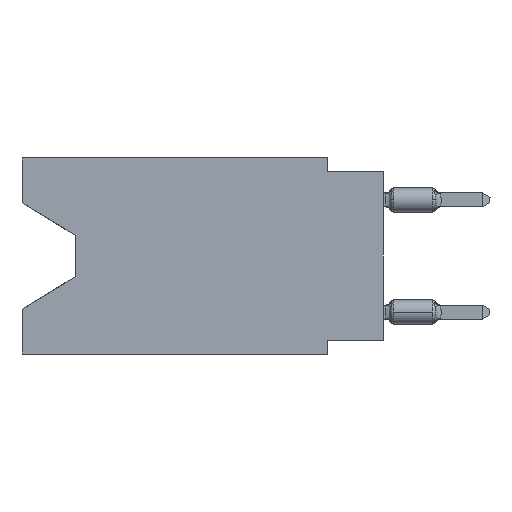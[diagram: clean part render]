
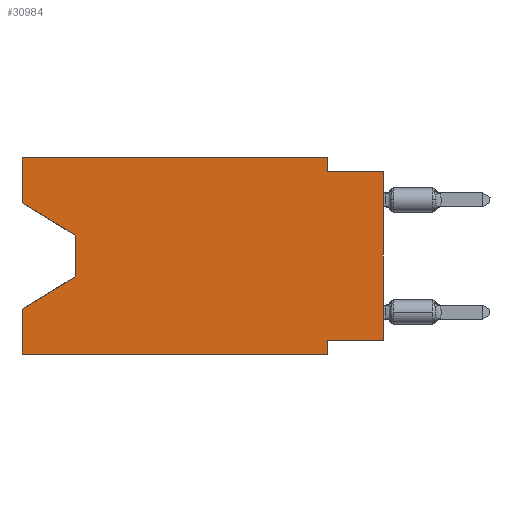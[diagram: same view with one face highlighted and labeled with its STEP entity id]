
A CAD part, left-side view. The second image highlights one B-rep face of the part: STEP entity #30984.
In plain terms, the highlighted planar face has unit normal (-1, 0, 0).
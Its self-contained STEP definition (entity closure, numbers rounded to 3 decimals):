
#1285 = VERTEX_POINT ( 'NONE', #12462 ) ;
#3430 = CARTESIAN_POINT ( 'NONE',  ( 0., 16.383, 0. ) ) ;
#3549 = VERTEX_POINT ( 'NONE', #6549 ) ;
#4236 = VERTEX_POINT ( 'NONE', #45789 ) ;
#4736 = DIRECTION ( 'NONE',  ( 0., -1., 0. ) ) ;
#6002 = CARTESIAN_POINT ( 'NONE',  ( 0., 16.383, 0. ) ) ;
#6549 = CARTESIAN_POINT ( 'NONE',  ( 0., 2.54, -8.89 ) ) ;
#6741 = ORIENTED_EDGE ( 'NONE', *, *, #22903, .F. ) ;
#6916 = LINE ( 'NONE', #33913, #56419 ) ;
#7163 = ORIENTED_EDGE ( 'NONE', *, *, #11240, .T. ) ;
#7805 = EDGE_CURVE ( 'NONE', #14312, #40535, #52317, .T. ) ;
#7838 = DIRECTION ( 'NONE',  ( 0., -1., 0. ) ) ;
#7940 = VECTOR ( 'NONE', #47661, 1000. ) ;
#7966 = ORIENTED_EDGE ( 'NONE', *, *, #21725, .T. ) ;
#8122 = CARTESIAN_POINT ( 'NONE',  ( 0., 16.383, -8.89 ) ) ;
#8151 = VECTOR ( 'NONE', #15307, 1000. ) ;
#8404 = ORIENTED_EDGE ( 'NONE', *, *, #32919, .F. ) ;
#9423 = DIRECTION ( 'NONE',  ( 0., 0., -1. ) ) ;
#9723 = LINE ( 'NONE', #51548, #49318 ) ;
#10751 = DIRECTION ( 'NONE',  ( 1., 0., 0. ) ) ;
#11240 = EDGE_CURVE ( 'NONE', #54903, #12754, #9723, .T. ) ;
#12462 = CARTESIAN_POINT ( 'NONE',  ( 0., 16.383, -8.89 ) ) ;
#12672 = LINE ( 'NONE', #21169, #59723 ) ;
#12754 = VERTEX_POINT ( 'NONE', #35183 ) ;
#13135 = AXIS2_PLACEMENT_3D ( 'NONE', #34107, #10751, #29230 ) ;
#14236 = ORIENTED_EDGE ( 'NONE', *, *, #34573, .T. ) ;
#14312 = VERTEX_POINT ( 'NONE', #44828 ) ;
#14423 = EDGE_CURVE ( 'NONE', #54903, #18775, #44248, .T. ) ;
#14842 = CARTESIAN_POINT ( 'NONE',  ( 0., 13.97, -5.385 ) ) ;
#14859 = CARTESIAN_POINT ( 'NONE',  ( 0., 0., -0.635 ) ) ;
#15307 = DIRECTION ( 'NONE',  ( 0., 1., 0. ) ) ;
#16430 = EDGE_CURVE ( 'NONE', #1285, #4236, #48883, .T. ) ;
#16643 = CARTESIAN_POINT ( 'NONE',  ( 0., 16.383, 0. ) ) ;
#18086 = VECTOR ( 'NONE', #9423, 1000. ) ;
#18430 = CARTESIAN_POINT ( 'NONE',  ( 0., 16.383, -2.038 ) ) ;
#18775 = VERTEX_POINT ( 'NONE', #6002 ) ;
#19167 = CARTESIAN_POINT ( 'NONE',  ( 0., 0., 0. ) ) ;
#19642 = EDGE_CURVE ( 'NONE', #41172, #4236, #29483, .T. ) ;
#19706 = ORIENTED_EDGE ( 'NONE', *, *, #16430, .F. ) ;
#19819 = FACE_OUTER_BOUND ( 'NONE', #45576, .T. ) ;
#20062 = LINE ( 'NONE', #19167, #59772 ) ;
#20123 = VERTEX_POINT ( 'NONE', #14859 ) ;
#21169 = CARTESIAN_POINT ( 'NONE',  ( 0., 0., -0.635 ) ) ;
#21725 = EDGE_CURVE ( 'NONE', #12754, #41172, #6916, .T. ) ;
#22335 = LINE ( 'NONE', #8122, #50082 ) ;
#22903 = EDGE_CURVE ( 'NONE', #47181, #47933, #29241, .T. ) ;
#23649 = CARTESIAN_POINT ( 'NONE',  ( 0., 2.54, -8.89 ) ) ;
#24770 = VECTOR ( 'NONE', #30599, 1000. ) ;
#26229 = CARTESIAN_POINT ( 'NONE',  ( 0., 0., -8.255 ) ) ;
#28644 = PLANE ( 'NONE',  #13135 ) ;
#28694 = DIRECTION ( 'NONE',  ( 0., 0., -1. ) ) ;
#28879 = VECTOR ( 'NONE', #4736, 1000. ) ;
#29230 = DIRECTION ( 'NONE',  ( 0., 0., -1. ) ) ;
#29241 = LINE ( 'NONE', #33820, #8151 ) ;
#29483 = LINE ( 'NONE', #33759, #7940 ) ;
#30599 = DIRECTION ( 'NONE',  ( 0., 0., 1. ) ) ;
#30984 = ADVANCED_FACE ( 'NONE', ( #19819 ), #28644, .F. ) ;
#31453 = DIRECTION ( 'NONE',  ( 0., -1., 0. ) ) ;
#32006 = LINE ( 'NONE', #55057, #28879 ) ;
#32919 = EDGE_CURVE ( 'NONE', #47933, #3549, #50940, .T. ) ;
#33651 = CARTESIAN_POINT ( 'NONE',  ( 0., 2.54, -8.255 ) ) ;
#33759 = CARTESIAN_POINT ( 'NONE',  ( 0., 13.97, -5.385 ) ) ;
#33820 = CARTESIAN_POINT ( 'NONE',  ( 0., 0., -8.255 ) ) ;
#33913 = CARTESIAN_POINT ( 'NONE',  ( 0., 13.97, -3.505 ) ) ;
#34107 = CARTESIAN_POINT ( 'NONE',  ( 0., 16.383, 0. ) ) ;
#34563 = ORIENTED_EDGE ( 'NONE', *, *, #7805, .F. ) ;
#34573 = EDGE_CURVE ( 'NONE', #1285, #3549, #22335, .T. ) ;
#35183 = CARTESIAN_POINT ( 'NONE',  ( 0., 13.97, -3.505 ) ) ;
#35537 = VECTOR ( 'NONE', #28694, 1000. ) ;
#36615 = ORIENTED_EDGE ( 'NONE', *, *, #49183, .T. ) ;
#37982 = DIRECTION ( 'NONE',  ( 0., 0., 1. ) ) ;
#40095 = EDGE_CURVE ( 'NONE', #40535, #20123, #12672, .T. ) ;
#40535 = VERTEX_POINT ( 'NONE', #59812 ) ;
#41172 = VERTEX_POINT ( 'NONE', #14842 ) ;
#43289 = DIRECTION ( 'NONE',  ( 0., 0., -1. ) ) ;
#44248 = LINE ( 'NONE', #16643, #24770 ) ;
#44551 = ORIENTED_EDGE ( 'NONE', *, *, #40095, .F. ) ;
#44828 = CARTESIAN_POINT ( 'NONE',  ( 0., 2.54, 0. ) ) ;
#45576 = EDGE_LOOP ( 'NONE', ( #7163, #7966, #59653, #19706, #14236, #8404, #6741, #36615, #44551, #34563, #54943, #55765 ) ) ;
#45783 = DIRECTION ( 'NONE',  ( 0., -0.855, -0.519 ) ) ;
#45789 = CARTESIAN_POINT ( 'NONE',  ( 0., 16.383, -6.852 ) ) ;
#47181 = VERTEX_POINT ( 'NONE', #26229 ) ;
#47661 = DIRECTION ( 'NONE',  ( 0., 0.855, -0.519 ) ) ;
#47933 = VERTEX_POINT ( 'NONE', #33651 ) ;
#48315 = VECTOR ( 'NONE', #53166, 1000. ) ;
#48883 = LINE ( 'NONE', #3430, #48315 ) ;
#49183 = EDGE_CURVE ( 'NONE', #47181, #20123, #20062, .T. ) ;
#49318 = VECTOR ( 'NONE', #45783, 1000. ) ;
#49824 = EDGE_CURVE ( 'NONE', #18775, #14312, #32006, .T. ) ;
#50082 = VECTOR ( 'NONE', #31453, 1000. ) ;
#50940 = LINE ( 'NONE', #23649, #18086 ) ;
#51548 = CARTESIAN_POINT ( 'NONE',  ( 0., 16.383, -2.038 ) ) ;
#52317 = LINE ( 'NONE', #56904, #35537 ) ;
#53166 = DIRECTION ( 'NONE',  ( 0., 0., 1. ) ) ;
#54903 = VERTEX_POINT ( 'NONE', #18430 ) ;
#54943 = ORIENTED_EDGE ( 'NONE', *, *, #49824, .F. ) ;
#55057 = CARTESIAN_POINT ( 'NONE',  ( 0., 16.383, 0. ) ) ;
#55765 = ORIENTED_EDGE ( 'NONE', *, *, #14423, .F. ) ;
#56419 = VECTOR ( 'NONE', #43289, 1000. ) ;
#56904 = CARTESIAN_POINT ( 'NONE',  ( 0., 2.54, 0. ) ) ;
#59653 = ORIENTED_EDGE ( 'NONE', *, *, #19642, .T. ) ;
#59723 = VECTOR ( 'NONE', #7838, 1000. ) ;
#59772 = VECTOR ( 'NONE', #37982, 1000. ) ;
#59812 = CARTESIAN_POINT ( 'NONE',  ( 0., 2.54, -0.635 ) ) ;
